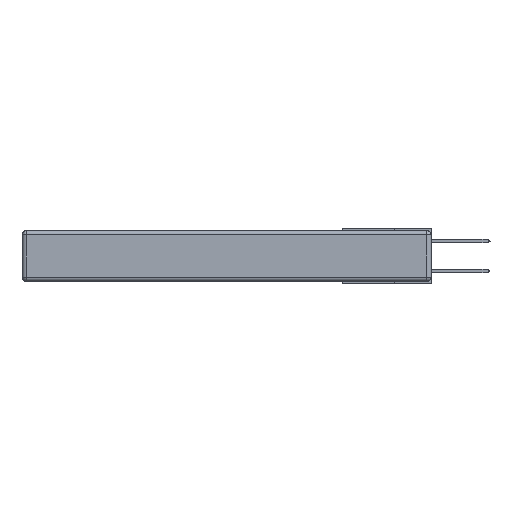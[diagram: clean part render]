
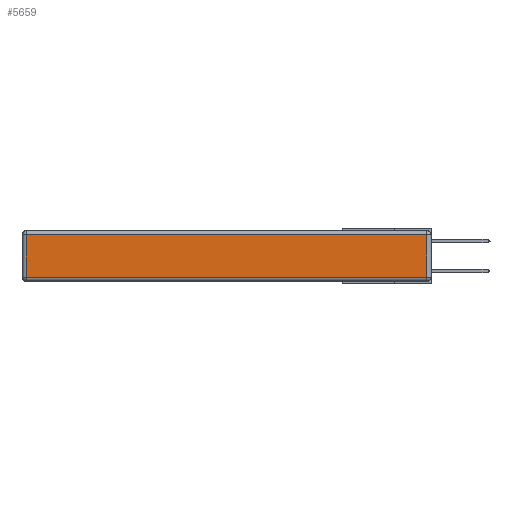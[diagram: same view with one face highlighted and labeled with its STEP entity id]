
A CAD part, left-side view. The second image highlights one B-rep face of the part: STEP entity #5659.
In plain terms, the highlighted planar face has unit normal (-1, 0, 0).
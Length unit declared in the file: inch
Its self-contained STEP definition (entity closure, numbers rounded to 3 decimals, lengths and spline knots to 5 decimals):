
#604 = CARTESIAN_POINT ( 'NONE',  ( 0., 2.75, -0.03 ) ) ;
#2663 = DIRECTION ( 'NONE',  ( 0., 0., 1. ) ) ;
#3063 = VECTOR ( 'NONE', #2663, 39.37008 ) ;
#3161 = ORIENTED_EDGE ( 'NONE', *, *, #23045, .T. ) ;
#4140 = AXIS2_PLACEMENT_3D ( 'NONE', #23604, #23696, #19520 ) ;
#4184 = CARTESIAN_POINT ( 'NONE',  ( 0., 0., -0.313 ) ) ;
#4221 = PLANE ( 'NONE',  #4140 ) ;
#4366 = DIRECTION ( 'NONE',  ( 0., -1., 0. ) ) ;
#5611 = ORIENTED_EDGE ( 'NONE', *, *, #14021, .T. ) ;
#5659 = ADVANCED_FACE ( 'NONE', ( #11433 ), #4221, .T. ) ;
#5819 = LINE ( 'NONE', #604, #7493 ) ;
#5826 = LINE ( 'NONE', #6267, #27384 ) ;
#6007 = DIRECTION ( 'NONE',  ( 0., 0., -1. ) ) ;
#6267 = CARTESIAN_POINT ( 'NONE',  ( 0., 2.72, -0.343 ) ) ;
#6885 = DIRECTION ( 'NONE',  ( 0., 1., 0. ) ) ;
#7493 = VECTOR ( 'NONE', #6885, 39.37008 ) ;
#7834 = CARTESIAN_POINT ( 'NONE',  ( 0., 0.03, -0.03 ) ) ;
#8460 = CARTESIAN_POINT ( 'NONE',  ( 0., 0.03, -0.313 ) ) ;
#10721 = ORIENTED_EDGE ( 'NONE', *, *, #24261, .T. ) ;
#10751 = VERTEX_POINT ( 'NONE', #24057 ) ;
#11433 = FACE_OUTER_BOUND ( 'NONE', #14606, .T. ) ;
#12971 = VECTOR ( 'NONE', #4366, 39.37008 ) ;
#13790 = VERTEX_POINT ( 'NONE', #7834 ) ;
#14021 = EDGE_CURVE ( 'NONE', #13790, #26753, #5819, .T. ) ;
#14606 = EDGE_LOOP ( 'NONE', ( #3161, #18472, #5611, #10721 ) ) ;
#17728 = CARTESIAN_POINT ( 'NONE',  ( 0., 0.03, -0.343 ) ) ;
#18472 = ORIENTED_EDGE ( 'NONE', *, *, #24181, .T. ) ;
#19520 = DIRECTION ( 'NONE',  ( 0., 0., 1. ) ) ;
#20884 = LINE ( 'NONE', #4184, #12971 ) ;
#21141 = LINE ( 'NONE', #17728, #3063 ) ;
#21441 = VERTEX_POINT ( 'NONE', #8460 ) ;
#23045 = EDGE_CURVE ( 'NONE', #10751, #21441, #20884, .T. ) ;
#23604 = CARTESIAN_POINT ( 'NONE',  ( 0., 0., -0.343 ) ) ;
#23696 = DIRECTION ( 'NONE',  ( -1., 0., 0. ) ) ;
#24057 = CARTESIAN_POINT ( 'NONE',  ( 0., 2.72, -0.313 ) ) ;
#24181 = EDGE_CURVE ( 'NONE', #21441, #13790, #21141, .T. ) ;
#24261 = EDGE_CURVE ( 'NONE', #26753, #10751, #5826, .T. ) ;
#25795 = CARTESIAN_POINT ( 'NONE',  ( 0., 2.72, -0.03 ) ) ;
#26753 = VERTEX_POINT ( 'NONE', #25795 ) ;
#27384 = VECTOR ( 'NONE', #6007, 39.37008 ) ;
